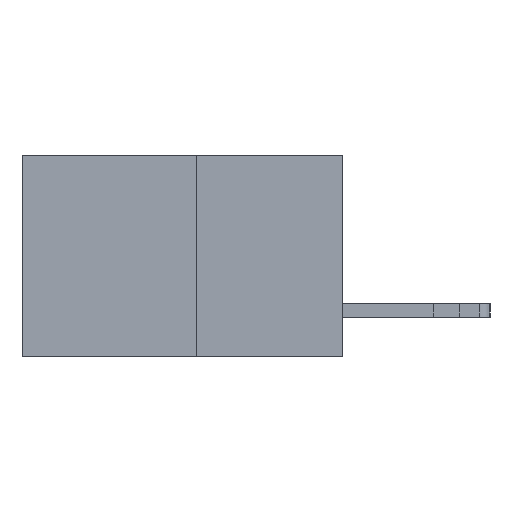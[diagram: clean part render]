
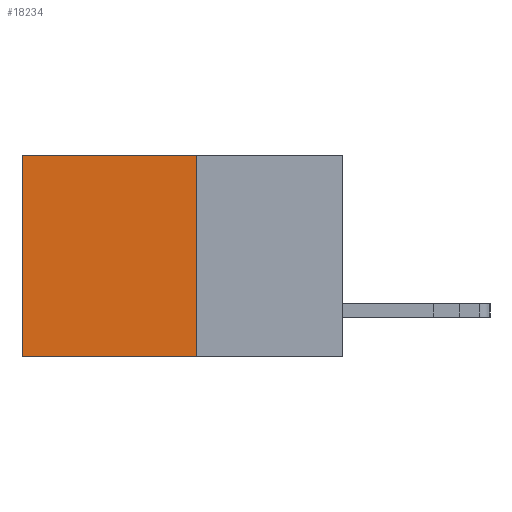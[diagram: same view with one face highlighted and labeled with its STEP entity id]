
A CAD part, left-side view. The second image highlights one B-rep face of the part: STEP entity #18234.
In plain terms, the highlighted planar face has unit normal (-1, 0, 0).
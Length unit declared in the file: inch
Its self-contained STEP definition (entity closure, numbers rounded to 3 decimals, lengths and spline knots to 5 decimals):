
#1191 = PLANE ( 'NONE',  #1767 ) ;
#1223 = CARTESIAN_POINT ( 'NONE',  ( 0.277, 0.27, 0. ) ) ;
#1767 = AXIS2_PLACEMENT_3D ( 'NONE', #3609, #20383, #6057 ) ;
#2072 = CARTESIAN_POINT ( 'NONE',  ( 0.277, 0.59, 0. ) ) ;
#3609 = CARTESIAN_POINT ( 'NONE',  ( 0.277, 0.27, -0.37 ) ) ;
#5250 = DIRECTION ( 'NONE',  ( 0., 1., 0. ) ) ;
#5292 = VECTOR ( 'NONE', #5558, 39.37008 ) ;
#5558 = DIRECTION ( 'NONE',  ( 0., 0., -1. ) ) ;
#5592 = ORIENTED_EDGE ( 'NONE', *, *, #23556, .F. ) ;
#6057 = DIRECTION ( 'NONE',  ( 0., 0., -1. ) ) ;
#8228 = CARTESIAN_POINT ( 'NONE',  ( 0.277, 0.27, -0.37 ) ) ;
#8256 = VERTEX_POINT ( 'NONE', #1223 ) ;
#8330 = DIRECTION ( 'NONE',  ( 0., 1., 0. ) ) ;
#8736 = ORIENTED_EDGE ( 'NONE', *, *, #22856, .F. ) ;
#9284 = LINE ( 'NONE', #23724, #27585 ) ;
#10190 = CARTESIAN_POINT ( 'NONE',  ( 0.277, 0.27, -0.37 ) ) ;
#11684 = LINE ( 'NONE', #29361, #5292 ) ;
#11701 = VERTEX_POINT ( 'NONE', #2072 ) ;
#11888 = EDGE_CURVE ( 'NONE', #8256, #11701, #29423, .T. ) ;
#12916 = CARTESIAN_POINT ( 'NONE',  ( 0.277, 0.59, -0.37 ) ) ;
#13310 = VERTEX_POINT ( 'NONE', #10190 ) ;
#13629 = FACE_OUTER_BOUND ( 'NONE', #20119, .T. ) ;
#14147 = DIRECTION ( 'NONE',  ( 0., 0., -1. ) ) ;
#15108 = ORIENTED_EDGE ( 'NONE', *, *, #11888, .T. ) ;
#16211 = VERTEX_POINT ( 'NONE', #12916 ) ;
#17174 = CARTESIAN_POINT ( 'NONE',  ( 0.277, 0.27, 0. ) ) ;
#18234 = ADVANCED_FACE ( 'NONE', ( #13629 ), #1191, .F. ) ;
#18368 = LINE ( 'NONE', #8228, #22437 ) ;
#20119 = EDGE_LOOP ( 'NONE', ( #26460, #5592, #8736, #15108 ) ) ;
#20383 = DIRECTION ( 'NONE',  ( 1., 0., 0. ) ) ;
#22351 = VECTOR ( 'NONE', #5250, 39.37008 ) ;
#22437 = VECTOR ( 'NONE', #8330, 39.37008 ) ;
#22856 = EDGE_CURVE ( 'NONE', #8256, #13310, #11684, .T. ) ;
#23556 = EDGE_CURVE ( 'NONE', #13310, #16211, #18368, .T. ) ;
#23724 = CARTESIAN_POINT ( 'NONE',  ( 0.277, 0.59, -0.37 ) ) ;
#26460 = ORIENTED_EDGE ( 'NONE', *, *, #29281, .T. ) ;
#27585 = VECTOR ( 'NONE', #14147, 39.37008 ) ;
#29281 = EDGE_CURVE ( 'NONE', #11701, #16211, #9284, .T. ) ;
#29361 = CARTESIAN_POINT ( 'NONE',  ( 0.277, 0.27, -0.37 ) ) ;
#29423 = LINE ( 'NONE', #17174, #22351 ) ;
